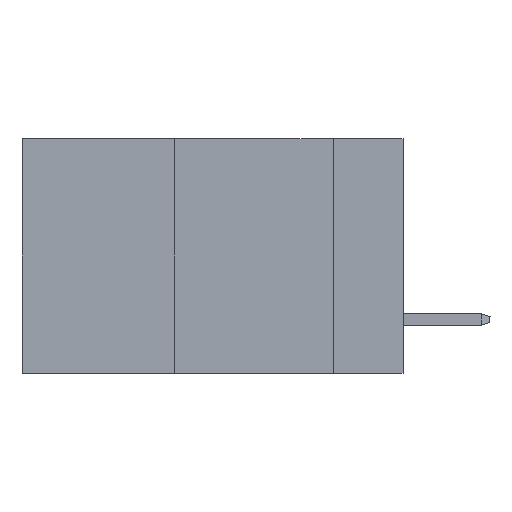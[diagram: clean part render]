
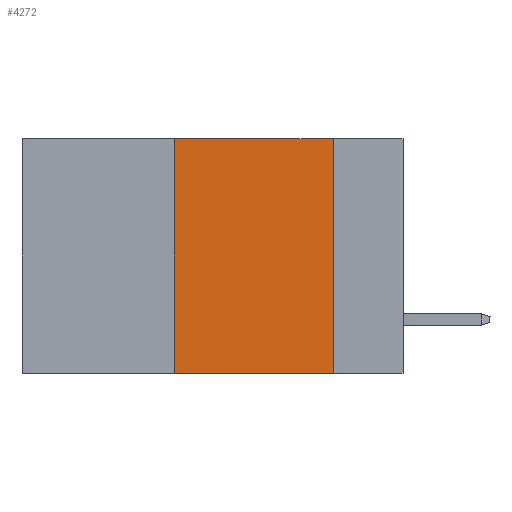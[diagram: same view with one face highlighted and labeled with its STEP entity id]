
A CAD part, left-side view. The second image highlights one B-rep face of the part: STEP entity #4272.
In plain terms, the highlighted planar face has unit normal (-1, 0, 0).
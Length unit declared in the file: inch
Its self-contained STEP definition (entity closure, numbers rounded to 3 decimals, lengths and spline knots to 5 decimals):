
#200 = DIRECTION ( 'NONE',  ( 0., -1., 0. ) ) ;
#699 = VERTEX_POINT ( 'NONE', #5038 ) ;
#802 = CARTESIAN_POINT ( 'NONE',  ( 0., 0.36, -0.37 ) ) ;
#1090 = LINE ( 'NONE', #2929, #1374 ) ;
#1374 = VECTOR ( 'NONE', #2109, 39.37008 ) ;
#2109 = DIRECTION ( 'NONE',  ( 0., -1., 0. ) ) ;
#2155 = CARTESIAN_POINT ( 'NONE',  ( 0., 0.11, -0.37 ) ) ;
#2929 = CARTESIAN_POINT ( 'NONE',  ( 0., 0.6, -0.37 ) ) ;
#3006 = EDGE_LOOP ( 'NONE', ( #9374, #9578, #6945, #11024 ) ) ;
#3285 = LINE ( 'NONE', #11448, #7201 ) ;
#3447 = EDGE_CURVE ( 'NONE', #12705, #8310, #9819, .T. ) ;
#3608 = CARTESIAN_POINT ( 'NONE',  ( 0., 0.36, 0. ) ) ;
#3726 = DIRECTION ( 'NONE',  ( 1., 0., 0. ) ) ;
#4272 = ADVANCED_FACE ( 'NONE', ( #6545 ), #8602, .F. ) ;
#4339 = EDGE_CURVE ( 'NONE', #699, #12705, #3285, .T. ) ;
#4744 = CARTESIAN_POINT ( 'NONE',  ( 0., 0.6, 0. ) ) ;
#5038 = CARTESIAN_POINT ( 'NONE',  ( 0., 0.36, 0. ) ) ;
#5673 = DIRECTION ( 'NONE',  ( 0., 0., 1. ) ) ;
#6545 = FACE_OUTER_BOUND ( 'NONE', #3006, .T. ) ;
#6945 = ORIENTED_EDGE ( 'NONE', *, *, #8992, .F. ) ;
#7201 = VECTOR ( 'NONE', #200, 39.37008 ) ;
#7757 = VECTOR ( 'NONE', #5673, 39.37008 ) ;
#7792 = DIRECTION ( 'NONE',  ( 0., 0., -1. ) ) ;
#8310 = VERTEX_POINT ( 'NONE', #2155 ) ;
#8602 = PLANE ( 'NONE',  #9997 ) ;
#8992 = EDGE_CURVE ( 'NONE', #9582, #699, #12766, .T. ) ;
#9374 = ORIENTED_EDGE ( 'NONE', *, *, #3447, .F. ) ;
#9578 = ORIENTED_EDGE ( 'NONE', *, *, #4339, .F. ) ;
#9582 = VERTEX_POINT ( 'NONE', #802 ) ;
#9819 = LINE ( 'NONE', #9939, #12550 ) ;
#9939 = CARTESIAN_POINT ( 'NONE',  ( 0., 0.11, 0. ) ) ;
#9997 = AXIS2_PLACEMENT_3D ( 'NONE', #4744, #3726, #7792 ) ;
#10882 = DIRECTION ( 'NONE',  ( 0., 0., -1. ) ) ;
#11024 = ORIENTED_EDGE ( 'NONE', *, *, #11936, .T. ) ;
#11448 = CARTESIAN_POINT ( 'NONE',  ( 0., 0.6, 0. ) ) ;
#11936 = EDGE_CURVE ( 'NONE', #9582, #8310, #1090, .T. ) ;
#11978 = CARTESIAN_POINT ( 'NONE',  ( 0., 0.11, 0. ) ) ;
#12550 = VECTOR ( 'NONE', #10882, 39.37008 ) ;
#12705 = VERTEX_POINT ( 'NONE', #11978 ) ;
#12766 = LINE ( 'NONE', #3608, #7757 ) ;
